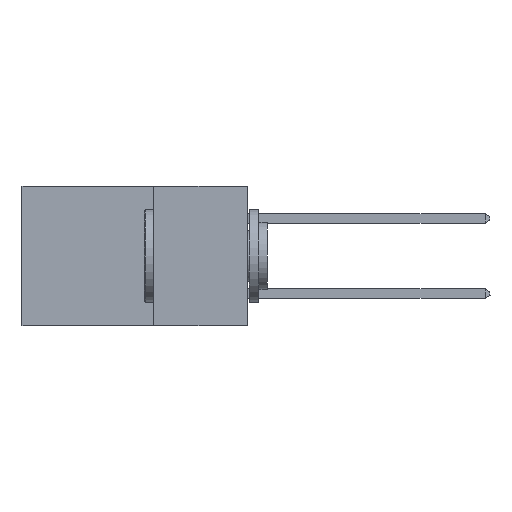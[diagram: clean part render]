
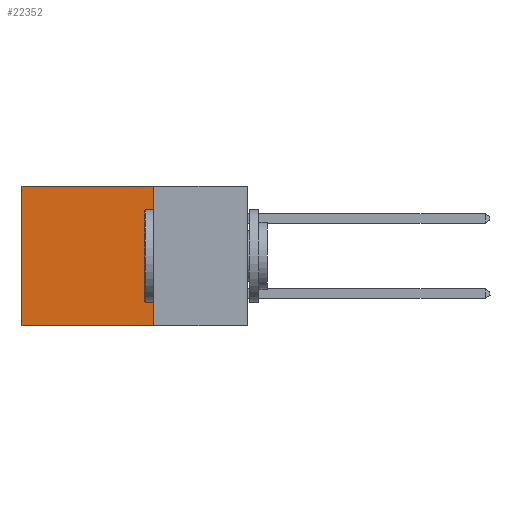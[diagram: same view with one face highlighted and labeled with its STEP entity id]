
A CAD part, left-side view. The second image highlights one B-rep face of the part: STEP entity #22352.
In plain terms, the highlighted planar face has unit normal (-1, 0, 0).
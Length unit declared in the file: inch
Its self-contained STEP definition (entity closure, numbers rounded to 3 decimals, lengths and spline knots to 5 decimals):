
#1488 = EDGE_LOOP ( 'NONE', ( #24850, #6405, #6113, #6882 ) ) ;
#1844 = DIRECTION ( 'NONE',  ( 0., 1., 0. ) ) ;
#3121 = VERTEX_POINT ( 'NONE', #22239 ) ;
#3965 = VERTEX_POINT ( 'NONE', #16902 ) ;
#4060 = DIRECTION ( 'NONE',  ( 1., 0., 0. ) ) ;
#4529 = CARTESIAN_POINT ( 'NONE',  ( 0.298, 0.25, -0.37 ) ) ;
#5543 = FACE_OUTER_BOUND ( 'NONE', #1488, .T. ) ;
#6113 = ORIENTED_EDGE ( 'NONE', *, *, #24073, .F. ) ;
#6405 = ORIENTED_EDGE ( 'NONE', *, *, #19578, .F. ) ;
#6490 = DIRECTION ( 'NONE',  ( 0., 1., 0. ) ) ;
#6882 = ORIENTED_EDGE ( 'NONE', *, *, #17529, .T. ) ;
#7781 = CARTESIAN_POINT ( 'NONE',  ( 0.298, 0.25, 0. ) ) ;
#7903 = PLANE ( 'NONE',  #13078 ) ;
#9621 = VERTEX_POINT ( 'NONE', #18651 ) ;
#9754 = CARTESIAN_POINT ( 'NONE',  ( 0.298, 0.6, 0. ) ) ;
#9863 = CARTESIAN_POINT ( 'NONE',  ( 0.298, 0.25, 0. ) ) ;
#9894 = DIRECTION ( 'NONE',  ( 0., 0., -1. ) ) ;
#10039 = DIRECTION ( 'NONE',  ( 0., 0., -1. ) ) ;
#10498 = LINE ( 'NONE', #9754, #17614 ) ;
#13078 = AXIS2_PLACEMENT_3D ( 'NONE', #16020, #4060, #9894 ) ;
#13187 = VECTOR ( 'NONE', #10039, 39.37008 ) ;
#14037 = CARTESIAN_POINT ( 'NONE',  ( 0.298, 0.25, -0.37 ) ) ;
#15736 = LINE ( 'NONE', #7781, #21730 ) ;
#16020 = CARTESIAN_POINT ( 'NONE',  ( 0.298, 0.25, 0. ) ) ;
#16902 = CARTESIAN_POINT ( 'NONE',  ( 0.298, 0.6, 0. ) ) ;
#17529 = EDGE_CURVE ( 'NONE', #3121, #3965, #15736, .T. ) ;
#17614 = VECTOR ( 'NONE', #24277, 39.37008 ) ;
#18651 = CARTESIAN_POINT ( 'NONE',  ( 0.298, 0.6, -0.37 ) ) ;
#19578 = EDGE_CURVE ( 'NONE', #20460, #9621, #20102, .T. ) ;
#20102 = LINE ( 'NONE', #4529, #23154 ) ;
#20460 = VERTEX_POINT ( 'NONE', #14037 ) ;
#21730 = VECTOR ( 'NONE', #1844, 39.37008 ) ;
#21826 = EDGE_CURVE ( 'NONE', #3965, #9621, #10498, .T. ) ;
#22239 = CARTESIAN_POINT ( 'NONE',  ( 0.298, 0.25, 0. ) ) ;
#22352 = ADVANCED_FACE ( 'NONE', ( #5543 ), #7903, .F. ) ;
#23154 = VECTOR ( 'NONE', #6490, 39.37008 ) ;
#23925 = LINE ( 'NONE', #9863, #13187 ) ;
#24073 = EDGE_CURVE ( 'NONE', #3121, #20460, #23925, .T. ) ;
#24277 = DIRECTION ( 'NONE',  ( 0., 0., -1. ) ) ;
#24850 = ORIENTED_EDGE ( 'NONE', *, *, #21826, .T. ) ;
